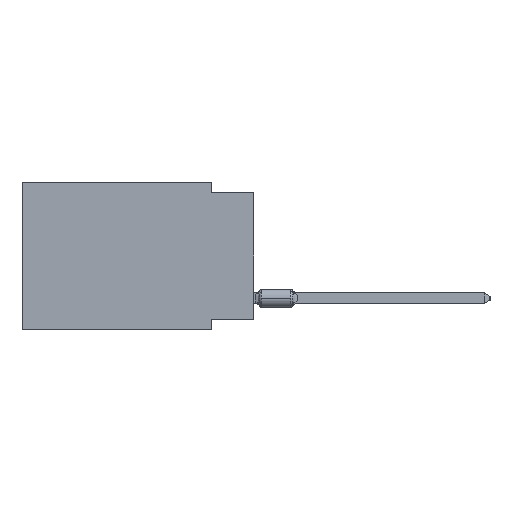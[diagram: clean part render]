
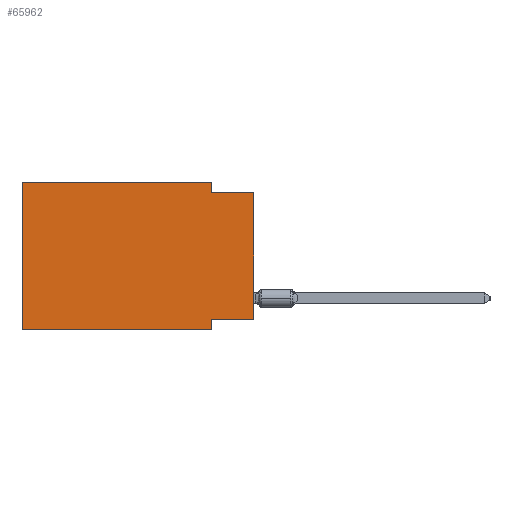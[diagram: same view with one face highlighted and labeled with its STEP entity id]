
A CAD part, left-side view. The second image highlights one B-rep face of the part: STEP entity #65962.
In plain terms, the highlighted planar face has unit normal (-1, 0, 0).
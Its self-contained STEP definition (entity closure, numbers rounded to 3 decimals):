
#243 = ORIENTED_EDGE ( 'NONE', *, *, #777, .F. ) ;
#777 = EDGE_CURVE ( 'NONE', #69633, #16685, #11913, .T. ) ;
#1591 = EDGE_CURVE ( 'NONE', #16685, #83610, #66951, .T. ) ;
#1623 = CARTESIAN_POINT ( 'NONE',  ( 0., 0., -0.635 ) ) ;
#7008 = LINE ( 'NONE', #65619, #26906 ) ;
#7754 = ORIENTED_EDGE ( 'NONE', *, *, #1591, .F. ) ;
#9090 = PLANE ( 'NONE',  #14405 ) ;
#10498 = CARTESIAN_POINT ( 'NONE',  ( 0., 13.97, 0. ) ) ;
#11469 = VERTEX_POINT ( 'NONE', #25600 ) ;
#11873 = CARTESIAN_POINT ( 'NONE',  ( 0., 13.97, 0. ) ) ;
#11913 = LINE ( 'NONE', #57285, #23593 ) ;
#12681 = VERTEX_POINT ( 'NONE', #11873 ) ;
#13778 = CARTESIAN_POINT ( 'NONE',  ( 0., 13.97, 0. ) ) ;
#14405 = AXIS2_PLACEMENT_3D ( 'NONE', #10498, #75738, #39315 ) ;
#16685 = VERTEX_POINT ( 'NONE', #55034 ) ;
#16696 = DIRECTION ( 'NONE',  ( 0., 0., 1. ) ) ;
#18056 = FACE_OUTER_BOUND ( 'NONE', #78653, .T. ) ;
#21169 = CARTESIAN_POINT ( 'NONE',  ( 0., 0., -8.255 ) ) ;
#22349 = VERTEX_POINT ( 'NONE', #26622 ) ;
#23593 = VECTOR ( 'NONE', #77634, 1000. ) ;
#25600 = CARTESIAN_POINT ( 'NONE',  ( 0., 2.54, -8.255 ) ) ;
#26476 = LINE ( 'NONE', #55327, #46077 ) ;
#26622 = CARTESIAN_POINT ( 'NONE',  ( 0., 13.97, -8.89 ) ) ;
#26906 = VECTOR ( 'NONE', #43390, 1000. ) ;
#27436 = EDGE_CURVE ( 'NONE', #62596, #11469, #44855, .T. ) ;
#28548 = EDGE_CURVE ( 'NONE', #22349, #59352, #87919, .T. ) ;
#29267 = CARTESIAN_POINT ( 'NONE',  ( 0., 13.97, 0. ) ) ;
#31168 = ORIENTED_EDGE ( 'NONE', *, *, #40064, .F. ) ;
#32107 = VECTOR ( 'NONE', #43895, 1000. ) ;
#32267 = ORIENTED_EDGE ( 'NONE', *, *, #27436, .F. ) ;
#32268 = VECTOR ( 'NONE', #58216, 1000. ) ;
#37423 = VECTOR ( 'NONE', #73245, 1000. ) ;
#39315 = DIRECTION ( 'NONE',  ( 0., 0., -1. ) ) ;
#40064 = EDGE_CURVE ( 'NONE', #12681, #69633, #86966, .T. ) ;
#42550 = ORIENTED_EDGE ( 'NONE', *, *, #28548, .T. ) ;
#43390 = DIRECTION ( 'NONE',  ( 0., 0., -1. ) ) ;
#43895 = DIRECTION ( 'NONE',  ( 0., -1., 0. ) ) ;
#43910 = CARTESIAN_POINT ( 'NONE',  ( 0., 0., -8.255 ) ) ;
#44855 = LINE ( 'NONE', #43910, #37423 ) ;
#45186 = EDGE_CURVE ( 'NONE', #22349, #12681, #78585, .T. ) ;
#46077 = VECTOR ( 'NONE', #16696, 1000. ) ;
#46726 = EDGE_CURVE ( 'NONE', #62596, #83610, #26476, .T. ) ;
#55034 = CARTESIAN_POINT ( 'NONE',  ( 0., 2.54, -0.635 ) ) ;
#55327 = CARTESIAN_POINT ( 'NONE',  ( 0., 0., 0. ) ) ;
#57177 = CARTESIAN_POINT ( 'NONE',  ( 0., 2.54, 0. ) ) ;
#57285 = CARTESIAN_POINT ( 'NONE',  ( 0., 2.54, 0. ) ) ;
#57443 = EDGE_CURVE ( 'NONE', #11469, #59352, #7008, .T. ) ;
#58216 = DIRECTION ( 'NONE',  ( 0., 0., 1. ) ) ;
#59352 = VERTEX_POINT ( 'NONE', #91460 ) ;
#61836 = ORIENTED_EDGE ( 'NONE', *, *, #45186, .F. ) ;
#62596 = VERTEX_POINT ( 'NONE', #21169 ) ;
#65619 = CARTESIAN_POINT ( 'NONE',  ( 0., 2.54, -8.89 ) ) ;
#65962 = ADVANCED_FACE ( 'NONE', ( #18056 ), #9090, .F. ) ;
#66951 = LINE ( 'NONE', #81635, #75092 ) ;
#67887 = DIRECTION ( 'NONE',  ( 0., -1., 0. ) ) ;
#69633 = VERTEX_POINT ( 'NONE', #57177 ) ;
#73245 = DIRECTION ( 'NONE',  ( 0., 1., 0. ) ) ;
#75092 = VECTOR ( 'NONE', #67887, 1000. ) ;
#75738 = DIRECTION ( 'NONE',  ( 1., 0., 0. ) ) ;
#77634 = DIRECTION ( 'NONE',  ( 0., 0., -1. ) ) ;
#78585 = LINE ( 'NONE', #13778, #32268 ) ;
#78653 = EDGE_LOOP ( 'NONE', ( #88644, #7754, #243, #31168, #61836, #42550, #92263, #32267 ) ) ;
#79904 = DIRECTION ( 'NONE',  ( 0., -1., 0. ) ) ;
#81635 = CARTESIAN_POINT ( 'NONE',  ( 0., 0., -0.635 ) ) ;
#83610 = VERTEX_POINT ( 'NONE', #1623 ) ;
#86966 = LINE ( 'NONE', #29267, #32107 ) ;
#86996 = CARTESIAN_POINT ( 'NONE',  ( 0., 13.97, -8.89 ) ) ;
#87919 = LINE ( 'NONE', #86996, #93486 ) ;
#88644 = ORIENTED_EDGE ( 'NONE', *, *, #46726, .T. ) ;
#91460 = CARTESIAN_POINT ( 'NONE',  ( 0., 2.54, -8.89 ) ) ;
#92263 = ORIENTED_EDGE ( 'NONE', *, *, #57443, .F. ) ;
#93486 = VECTOR ( 'NONE', #79904, 1000. ) ;
